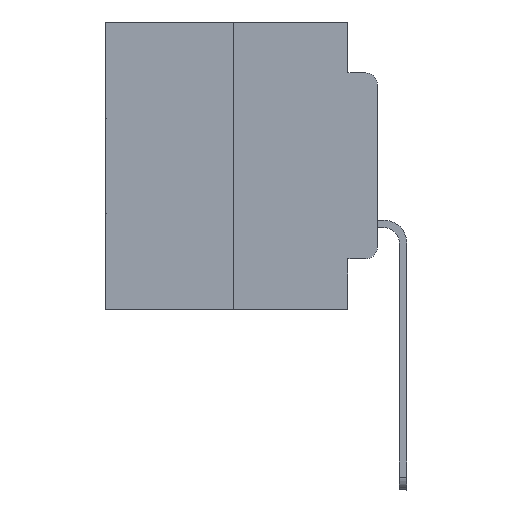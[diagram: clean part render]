
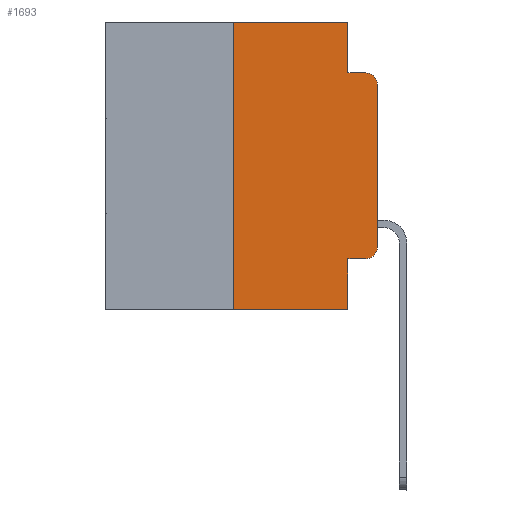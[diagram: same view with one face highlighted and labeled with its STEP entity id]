
A CAD part, left-side view. The second image highlights one B-rep face of the part: STEP entity #1693.
In plain terms, the highlighted planar face has unit normal (-1, 0, 0).
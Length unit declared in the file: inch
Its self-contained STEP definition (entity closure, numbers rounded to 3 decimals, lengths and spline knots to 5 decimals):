
#185 = EDGE_CURVE ( 'NONE', #16687, #4240, #28968, .T. ) ;
#373 = AXIS2_PLACEMENT_3D ( 'NONE', #15844, #24846, #8854 ) ;
#504 = CARTESIAN_POINT ( 'NONE',  ( 0., 0.473, -0.5 ) ) ;
#1060 = AXIS2_PLACEMENT_3D ( 'NONE', #18024, #11654, #6772 ) ;
#1243 = VECTOR ( 'NONE', #10314, 39.37008 ) ;
#1305 = VECTOR ( 'NONE', #3318, 39.37008 ) ;
#1471 = DIRECTION ( 'NONE',  ( 0., -1., 0. ) ) ;
#1626 = CARTESIAN_POINT ( 'NONE',  ( 0., 0.473, 0. ) ) ;
#1693 = ADVANCED_FACE ( 'NONE', ( #22759 ), #9294, .F. ) ;
#1765 = LINE ( 'NONE', #8991, #7613 ) ;
#2171 = EDGE_CURVE ( 'NONE', #20565, #18866, #23447, .T. ) ;
#2210 = AXIS2_PLACEMENT_3D ( 'NONE', #11397, #27103, #9023 ) ;
#2461 = CARTESIAN_POINT ( 'NONE',  ( 0., 0.02, -0.4115 ) ) ;
#3300 = CARTESIAN_POINT ( 'NONE',  ( 0., 0., -0.3915 ) ) ;
#3318 = DIRECTION ( 'NONE',  ( 0., 0., 1. ) ) ;
#3326 = CARTESIAN_POINT ( 'NONE',  ( 0., 0., -0.1085 ) ) ;
#3769 = VERTEX_POINT ( 'NONE', #3799 ) ;
#3799 = CARTESIAN_POINT ( 'NONE',  ( 0., 0.051, -0.5 ) ) ;
#3824 = VECTOR ( 'NONE', #1471, 39.37008 ) ;
#3933 = VERTEX_POINT ( 'NONE', #2461 ) ;
#4089 = ORIENTED_EDGE ( 'NONE', *, *, #28270, .F. ) ;
#4240 = VERTEX_POINT ( 'NONE', #22419 ) ;
#4604 = EDGE_LOOP ( 'NONE', ( #17345, #6834, #13711, #27670, #4089, #26941, #20596, #22196, #10031, #19162 ) ) ;
#5003 = VERTEX_POINT ( 'NONE', #28843 ) ;
#6772 = DIRECTION ( 'NONE',  ( 0., 0., -1. ) ) ;
#6834 = ORIENTED_EDGE ( 'NONE', *, *, #13822, .T. ) ;
#7613 = VECTOR ( 'NONE', #10776, 39.37008 ) ;
#8587 = LINE ( 'NONE', #12605, #8915 ) ;
#8854 = DIRECTION ( 'NONE',  ( 0., 0., -1. ) ) ;
#8915 = VECTOR ( 'NONE', #13041, 39.37008 ) ;
#8991 = CARTESIAN_POINT ( 'NONE',  ( 0., 0.051, 0. ) ) ;
#9023 = DIRECTION ( 'NONE',  ( 0., 0., -1. ) ) ;
#9294 = PLANE ( 'NONE',  #1060 ) ;
#10031 = ORIENTED_EDGE ( 'NONE', *, *, #29189, .T. ) ;
#10314 = DIRECTION ( 'NONE',  ( 0., 0., 1. ) ) ;
#10776 = DIRECTION ( 'NONE',  ( 0., 0., -1. ) ) ;
#11397 = CARTESIAN_POINT ( 'NONE',  ( 0., 0.02, -0.3915 ) ) ;
#11654 = DIRECTION ( 'NONE',  ( 1., 0., 0. ) ) ;
#11705 = VERTEX_POINT ( 'NONE', #20746 ) ;
#12118 = CIRCLE ( 'NONE', #2210, 0.02 ) ;
#12175 = EDGE_CURVE ( 'NONE', #3933, #20565, #12118, .T. ) ;
#12605 = CARTESIAN_POINT ( 'NONE',  ( 0., 0.051, 0. ) ) ;
#12719 = LINE ( 'NONE', #1626, #3824 ) ;
#13041 = DIRECTION ( 'NONE',  ( 0., 0., -1. ) ) ;
#13711 = ORIENTED_EDGE ( 'NONE', *, *, #185, .F. ) ;
#13822 = EDGE_CURVE ( 'NONE', #18866, #4240, #20685, .T. ) ;
#14740 = EDGE_CURVE ( 'NONE', #5003, #3769, #8587, .T. ) ;
#15844 = CARTESIAN_POINT ( 'NONE',  ( 0., 0.02, -0.1085 ) ) ;
#16576 = LINE ( 'NONE', #23928, #1243 ) ;
#16687 = VERTEX_POINT ( 'NONE', #18339 ) ;
#17105 = CARTESIAN_POINT ( 'NONE',  ( 0., 0.051, -0.4115 ) ) ;
#17345 = ORIENTED_EDGE ( 'NONE', *, *, #2171, .T. ) ;
#17591 = VECTOR ( 'NONE', #26127, 39.37008 ) ;
#18024 = CARTESIAN_POINT ( 'NONE',  ( 0., 0.473, 0. ) ) ;
#18339 = CARTESIAN_POINT ( 'NONE',  ( 0., 0.051, -0.0885 ) ) ;
#18580 = CARTESIAN_POINT ( 'NONE',  ( 0., 0., 0. ) ) ;
#18866 = VERTEX_POINT ( 'NONE', #3326 ) ;
#18954 = CARTESIAN_POINT ( 'NONE',  ( 0., 0.25, -0.5 ) ) ;
#19162 = ORIENTED_EDGE ( 'NONE', *, *, #12175, .T. ) ;
#20370 = EDGE_CURVE ( 'NONE', #20941, #3769, #23280, .T. ) ;
#20565 = VERTEX_POINT ( 'NONE', #3300 ) ;
#20596 = ORIENTED_EDGE ( 'NONE', *, *, #20370, .T. ) ;
#20685 = CIRCLE ( 'NONE', #373, 0.02 ) ;
#20746 = CARTESIAN_POINT ( 'NONE',  ( 0., 0.25, 0. ) ) ;
#20941 = VERTEX_POINT ( 'NONE', #18954 ) ;
#22174 = CARTESIAN_POINT ( 'NONE',  ( 0., 0.051, -0.0885 ) ) ;
#22196 = ORIENTED_EDGE ( 'NONE', *, *, #14740, .F. ) ;
#22419 = CARTESIAN_POINT ( 'NONE',  ( 0., 0.02, -0.0885 ) ) ;
#22759 = FACE_OUTER_BOUND ( 'NONE', #4604, .T. ) ;
#22768 = CARTESIAN_POINT ( 'NONE',  ( 0., 0.051, 0. ) ) ;
#23280 = LINE ( 'NONE', #504, #24709 ) ;
#23447 = LINE ( 'NONE', #18580, #1305 ) ;
#23928 = CARTESIAN_POINT ( 'NONE',  ( 0., 0.25, 0. ) ) ;
#24709 = VECTOR ( 'NONE', #24935, 39.37008 ) ;
#24846 = DIRECTION ( 'NONE',  ( -1., 0., 0. ) ) ;
#24935 = DIRECTION ( 'NONE',  ( 0., -1., 0. ) ) ;
#25353 = VERTEX_POINT ( 'NONE', #22768 ) ;
#25418 = EDGE_CURVE ( 'NONE', #20941, #11705, #16576, .T. ) ;
#26127 = DIRECTION ( 'NONE',  ( 0., -1., 0. ) ) ;
#26332 = DIRECTION ( 'NONE',  ( 0., -1., 0. ) ) ;
#26941 = ORIENTED_EDGE ( 'NONE', *, *, #25418, .F. ) ;
#27103 = DIRECTION ( 'NONE',  ( -1., 0., 0. ) ) ;
#27670 = ORIENTED_EDGE ( 'NONE', *, *, #28455, .F. ) ;
#27836 = VECTOR ( 'NONE', #26332, 39.37008 ) ;
#27888 = LINE ( 'NONE', #17105, #17591 ) ;
#28270 = EDGE_CURVE ( 'NONE', #11705, #25353, #12719, .T. ) ;
#28455 = EDGE_CURVE ( 'NONE', #25353, #16687, #1765, .T. ) ;
#28843 = CARTESIAN_POINT ( 'NONE',  ( 0., 0.051, -0.4115 ) ) ;
#28968 = LINE ( 'NONE', #22174, #27836 ) ;
#29189 = EDGE_CURVE ( 'NONE', #5003, #3933, #27888, .T. ) ;
